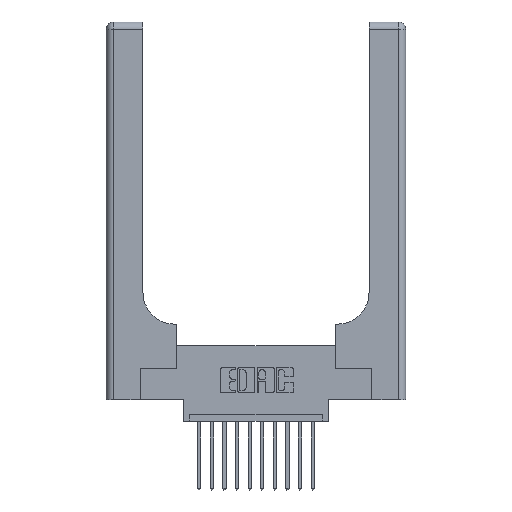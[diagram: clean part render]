
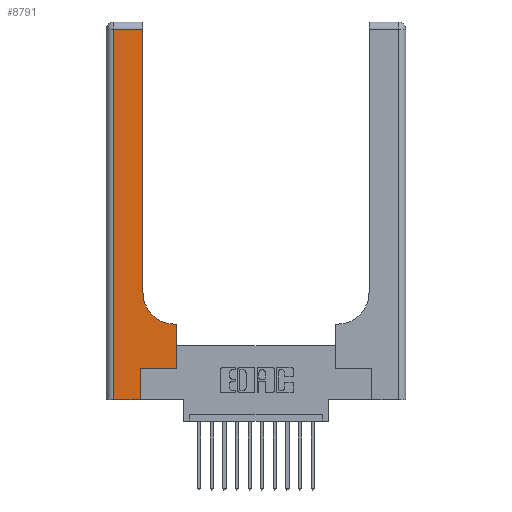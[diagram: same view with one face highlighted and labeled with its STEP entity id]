
A CAD part, top view. The second image highlights one B-rep face of the part: STEP entity #8791.
In plain terms, the highlighted planar face has unit normal (0, 0, 1).
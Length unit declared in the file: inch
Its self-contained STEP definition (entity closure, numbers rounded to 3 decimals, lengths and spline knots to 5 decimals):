
#104 = LINE ( 'NONE', #11329, #13774 ) ;
#172 = VECTOR ( 'NONE', #10302, 39.37008 ) ;
#292 = CARTESIAN_POINT ( 'NONE',  ( 0.269, 0.25, 0.37 ) ) ;
#900 = DIRECTION ( 'NONE',  ( 0., 1., 0. ) ) ;
#1276 = ORIENTED_EDGE ( 'NONE', *, *, #14289, .T. ) ;
#1671 = ORIENTED_EDGE ( 'NONE', *, *, #13665, .T. ) ;
#1728 = CARTESIAN_POINT ( 'NONE',  ( 0.2915, 2.94, 0.37 ) ) ;
#2081 = VERTEX_POINT ( 'NONE', #1728 ) ;
#2241 = ORIENTED_EDGE ( 'NONE', *, *, #15674, .T. ) ;
#2549 = DIRECTION ( 'NONE',  ( 1., 0., 0. ) ) ;
#2877 = CARTESIAN_POINT ( 'NONE',  ( 0.06, 0., 0.37 ) ) ;
#2966 = LINE ( 'NONE', #11900, #14959 ) ;
#3001 = CARTESIAN_POINT ( 'NONE',  ( 0.5415, 0.6, 0.37 ) ) ;
#3427 = CARTESIAN_POINT ( 'NONE',  ( 0.06, 3., 0.37 ) ) ;
#3467 = CARTESIAN_POINT ( 'NONE',  ( 0.269, 0., 0.37 ) ) ;
#3742 = CARTESIAN_POINT ( 'NONE',  ( 0.5415, 0.85, 0.37 ) ) ;
#3938 = DIRECTION ( 'NONE',  ( -1., 0., 0. ) ) ;
#4421 = DIRECTION ( 'NONE',  ( 0., 1., 0. ) ) ;
#4686 = FACE_OUTER_BOUND ( 'NONE', #8294, .T. ) ;
#4789 = PLANE ( 'NONE',  #5978 ) ;
#4790 = VERTEX_POINT ( 'NONE', #3467 ) ;
#4812 = VECTOR ( 'NONE', #2549, 39.37008 ) ;
#4970 = VECTOR ( 'NONE', #900, 39.37008 ) ;
#5392 = ORIENTED_EDGE ( 'NONE', *, *, #13046, .T. ) ;
#5978 = AXIS2_PLACEMENT_3D ( 'NONE', #7480, #12626, #14082 ) ;
#6462 = LINE ( 'NONE', #15193, #8546 ) ;
#7480 = CARTESIAN_POINT ( 'NONE',  ( 0., 3., 0.37 ) ) ;
#7556 = ORIENTED_EDGE ( 'NONE', *, *, #12230, .T. ) ;
#7564 = CARTESIAN_POINT ( 'NONE',  ( 0.2915, 0.85, 0.37 ) ) ;
#7640 = VERTEX_POINT ( 'NONE', #292 ) ;
#7973 = LINE ( 'NONE', #14291, #4812 ) ;
#8132 = EDGE_CURVE ( 'NONE', #12197, #16362, #14264, .T. ) ;
#8294 = EDGE_LOOP ( 'NONE', ( #7556, #2241, #13867, #15625, #14769, #1671, #5392, #11452, #1276 ) ) ;
#8546 = VECTOR ( 'NONE', #4421, 39.37008 ) ;
#8634 = DIRECTION ( 'NONE',  ( 1., 0., 0. ) ) ;
#8791 = ADVANCED_FACE ( 'NONE', ( #4686 ), #4789, .F. ) ;
#9112 = CARTESIAN_POINT ( 'NONE',  ( 0., 2.94, 0.37 ) ) ;
#9296 = VERTEX_POINT ( 'NONE', #7564 ) ;
#9297 = CARTESIAN_POINT ( 'NONE',  ( 0.06, 2.94, 0.37 ) ) ;
#10210 = LINE ( 'NONE', #12040, #13546 ) ;
#10302 = DIRECTION ( 'NONE',  ( 0., -1., 0. ) ) ;
#10659 = EDGE_CURVE ( 'NONE', #16766, #10865, #10210, .T. ) ;
#10865 = VERTEX_POINT ( 'NONE', #3001 ) ;
#11043 = EDGE_CURVE ( 'NONE', #4790, #7640, #6462, .T. ) ;
#11296 = CARTESIAN_POINT ( 'NONE',  ( 0.5585, 0.25, 0.37 ) ) ;
#11329 = CARTESIAN_POINT ( 'NONE',  ( 0., 0., 0.37 ) ) ;
#11452 = ORIENTED_EDGE ( 'NONE', *, *, #10659, .T. ) ;
#11725 = LINE ( 'NONE', #9112, #13781 ) ;
#11900 = CARTESIAN_POINT ( 'NONE',  ( 0.2915, 3., 0.37 ) ) ;
#12040 = CARTESIAN_POINT ( 'NONE',  ( 0.2915, 0.6, 0.37 ) ) ;
#12058 = LINE ( 'NONE', #11296, #4970 ) ;
#12197 = VERTEX_POINT ( 'NONE', #9297 ) ;
#12230 = EDGE_CURVE ( 'NONE', #9296, #2081, #2966, .T. ) ;
#12626 = DIRECTION ( 'NONE',  ( 0., 0., -1. ) ) ;
#12919 = CARTESIAN_POINT ( 'NONE',  ( 0.5585, 0.6, 0.37 ) ) ;
#13046 = EDGE_CURVE ( 'NONE', #13096, #16766, #12058, .T. ) ;
#13096 = VERTEX_POINT ( 'NONE', #14311 ) ;
#13145 = DIRECTION ( 'NONE',  ( 0., 1., 0. ) ) ;
#13518 = EDGE_CURVE ( 'NONE', #16362, #4790, #104, .T. ) ;
#13546 = VECTOR ( 'NONE', #14519, 39.37008 ) ;
#13665 = EDGE_CURVE ( 'NONE', #7640, #13096, #7973, .T. ) ;
#13774 = VECTOR ( 'NONE', #8634, 39.37008 ) ;
#13781 = VECTOR ( 'NONE', #3938, 39.37008 ) ;
#13867 = ORIENTED_EDGE ( 'NONE', *, *, #8132, .T. ) ;
#14046 = DIRECTION ( 'NONE',  ( 0., 0., -1. ) ) ;
#14082 = DIRECTION ( 'NONE',  ( -1., 0., 0. ) ) ;
#14264 = LINE ( 'NONE', #3427, #172 ) ;
#14289 = EDGE_CURVE ( 'NONE', #10865, #9296, #16499, .T. ) ;
#14291 = CARTESIAN_POINT ( 'NONE',  ( 0.269, 0.25, 0.37 ) ) ;
#14311 = CARTESIAN_POINT ( 'NONE',  ( 0.5585, 0.25, 0.37 ) ) ;
#14519 = DIRECTION ( 'NONE',  ( -1., 0., 0. ) ) ;
#14769 = ORIENTED_EDGE ( 'NONE', *, *, #11043, .T. ) ;
#14959 = VECTOR ( 'NONE', #13145, 39.37008 ) ;
#15193 = CARTESIAN_POINT ( 'NONE',  ( 0.269, 0., 0.37 ) ) ;
#15406 = DIRECTION ( 'NONE',  ( 1., 0., 0. ) ) ;
#15625 = ORIENTED_EDGE ( 'NONE', *, *, #13518, .T. ) ;
#15674 = EDGE_CURVE ( 'NONE', #2081, #12197, #11725, .T. ) ;
#16014 = AXIS2_PLACEMENT_3D ( 'NONE', #3742, #14046, #15406 ) ;
#16362 = VERTEX_POINT ( 'NONE', #2877 ) ;
#16499 = CIRCLE ( 'NONE', #16014, 0.25 ) ;
#16766 = VERTEX_POINT ( 'NONE', #12919 ) ;
